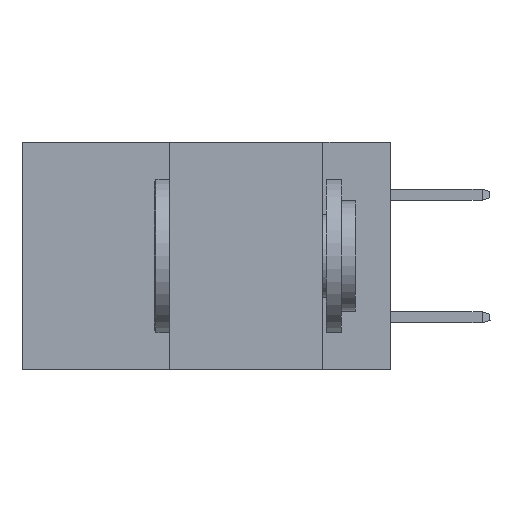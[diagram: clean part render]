
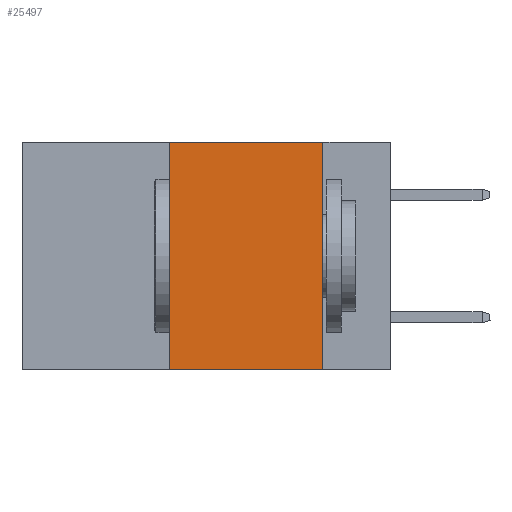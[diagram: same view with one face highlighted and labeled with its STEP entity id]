
A CAD part, left-side view. The second image highlights one B-rep face of the part: STEP entity #25497.
In plain terms, the highlighted planar face has unit normal (-1, 0, 0).
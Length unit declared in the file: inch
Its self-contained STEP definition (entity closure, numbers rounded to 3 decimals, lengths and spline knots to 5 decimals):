
#134 = VERTEX_POINT ( 'NONE', #13832 ) ;
#250 = CARTESIAN_POINT ( 'NONE',  ( 0., 0.6, 0. ) ) ;
#297 = FACE_OUTER_BOUND ( 'NONE', #25974, .T. ) ;
#926 = CARTESIAN_POINT ( 'NONE',  ( 0., 0.6, -0.37 ) ) ;
#1528 = VECTOR ( 'NONE', #23010, 39.37008 ) ;
#2549 = ORIENTED_EDGE ( 'NONE', *, *, #9788, .F. ) ;
#3101 = CARTESIAN_POINT ( 'NONE',  ( 0., 0.36, -0.37 ) ) ;
#3513 = DIRECTION ( 'NONE',  ( 0., 0., 1. ) ) ;
#4311 = DIRECTION ( 'NONE',  ( 1., 0., 0. ) ) ;
#6904 = PLANE ( 'NONE',  #26658 ) ;
#7469 = EDGE_CURVE ( 'NONE', #14215, #14576, #12669, .T. ) ;
#9788 = EDGE_CURVE ( 'NONE', #14576, #23403, #14938, .T. ) ;
#12069 = CARTESIAN_POINT ( 'NONE',  ( 0., 0.11, 0. ) ) ;
#12669 = LINE ( 'NONE', #23379, #17182 ) ;
#13275 = DIRECTION ( 'NONE',  ( 0., 0., -1. ) ) ;
#13832 = CARTESIAN_POINT ( 'NONE',  ( 0., 0.11, -0.37 ) ) ;
#14215 = VERTEX_POINT ( 'NONE', #3101 ) ;
#14385 = VECTOR ( 'NONE', #21660, 39.37008 ) ;
#14576 = VERTEX_POINT ( 'NONE', #23735 ) ;
#14938 = LINE ( 'NONE', #16040, #23241 ) ;
#15171 = ORIENTED_EDGE ( 'NONE', *, *, #22028, .T. ) ;
#16040 = CARTESIAN_POINT ( 'NONE',  ( 0., 0.6, 0. ) ) ;
#17182 = VECTOR ( 'NONE', #3513, 39.37008 ) ;
#19532 = LINE ( 'NONE', #12069, #1528 ) ;
#21660 = DIRECTION ( 'NONE',  ( 0., -1., 0. ) ) ;
#22028 = EDGE_CURVE ( 'NONE', #14215, #134, #24737, .T. ) ;
#22296 = CARTESIAN_POINT ( 'NONE',  ( 0., 0.11, 0. ) ) ;
#22564 = EDGE_CURVE ( 'NONE', #23403, #134, #19532, .T. ) ;
#23010 = DIRECTION ( 'NONE',  ( 0., 0., -1. ) ) ;
#23241 = VECTOR ( 'NONE', #24649, 39.37008 ) ;
#23253 = ORIENTED_EDGE ( 'NONE', *, *, #7469, .F. ) ;
#23379 = CARTESIAN_POINT ( 'NONE',  ( 0., 0.36, 0. ) ) ;
#23403 = VERTEX_POINT ( 'NONE', #22296 ) ;
#23735 = CARTESIAN_POINT ( 'NONE',  ( 0., 0.36, 0. ) ) ;
#24525 = ORIENTED_EDGE ( 'NONE', *, *, #22564, .F. ) ;
#24649 = DIRECTION ( 'NONE',  ( 0., -1., 0. ) ) ;
#24737 = LINE ( 'NONE', #926, #14385 ) ;
#25497 = ADVANCED_FACE ( 'NONE', ( #297 ), #6904, .F. ) ;
#25974 = EDGE_LOOP ( 'NONE', ( #24525, #2549, #23253, #15171 ) ) ;
#26658 = AXIS2_PLACEMENT_3D ( 'NONE', #250, #4311, #13275 ) ;
